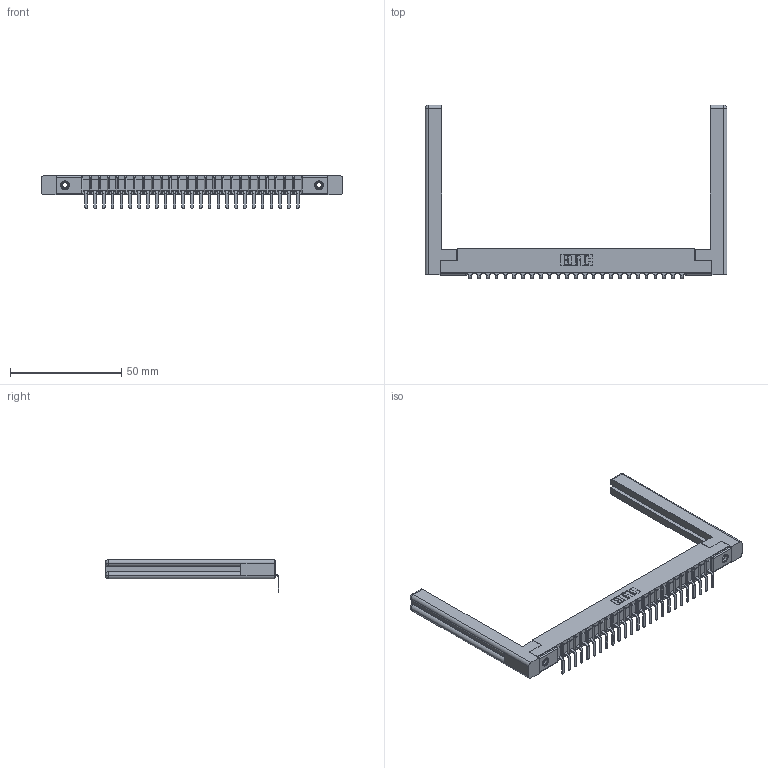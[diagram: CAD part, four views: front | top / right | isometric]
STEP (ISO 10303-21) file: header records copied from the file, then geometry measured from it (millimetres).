
FILE_DESCRIPTION (( 'STEP AP203' ), '1' );
FILE_NAME ('357-025-559-158.STEP', '2022-07-12T21:55:43', ( '' ), ( '' ), 'SwSTEP 2.0', 'SolidWorks 2020', '' );
FILE_SCHEMA (( 'CONFIG_CONTROL_DESIGN' ));
Length unit declared in the file: inch
Products named in the file (5): 307 Part_.156 Dia Mounting Holes; 345-250-001_345-250-001-102; 307-220-058; 357-025-559-158; 307-290-001_558 559 - 1 (Single)
Assembly tree (30 placements, depth 2):
  357-025-559-158
    307 Part_.156 Dia Mounting Holes
    307-290-001_558 559 - 1 (Single)  x25
    307-220-058  x2
    345-250-001_345-250-001-102  x2
Bounding box: 135.69 x 78.02 x 14.81 mm (x, y, z)
Volume: 16290.5 mm3; surface area: 18804.9 mm2
Topology: 30 solids, 30 shells, 1786 faces, 5027 edges, 3234 vertices
Faces by surface type: plane 1129, cylinder 581, sphere 52, torus 12, cone 12
Entity records: 26265 total; most frequent: CARTESIAN_POINT 4427, ORIENTED_EDGE 4352, DIRECTION 4276, EDGE_CURVE 2176, LINE 1658, VECTOR 1658, VERTEX_POINT 1406, AXIS2_PLACEMENT_3D 1309
